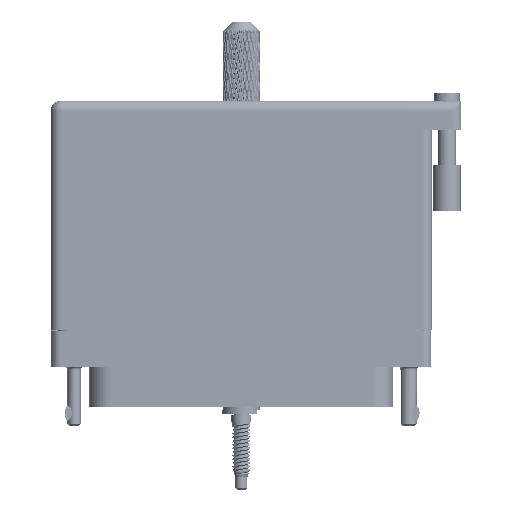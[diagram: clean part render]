
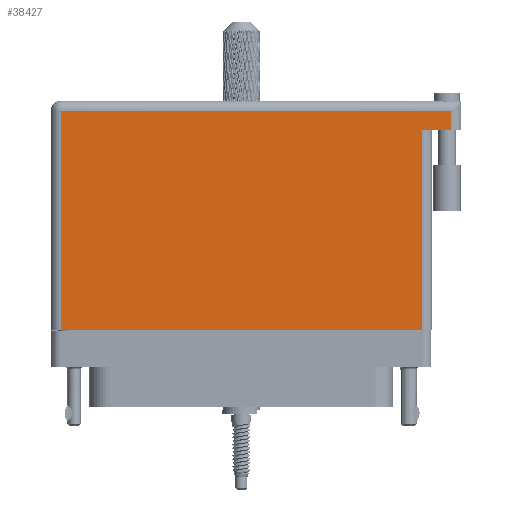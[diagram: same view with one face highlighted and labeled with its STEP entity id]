
A CAD part, front view. The second image highlights one B-rep face of the part: STEP entity #38427.
In plain terms, the highlighted face is planar.
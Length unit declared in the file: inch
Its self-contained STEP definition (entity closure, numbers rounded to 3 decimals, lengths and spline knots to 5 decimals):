
#741 = DIRECTION ( 'NONE',  ( -1., 0., 0. ) ) ;
#2738 = CARTESIAN_POINT ( 'NONE',  ( 1.43, 1.396, 0.4495 ) ) ;
#4744 = VECTOR ( 'NONE', #31527, 39.37008 ) ;
#10670 = EDGE_CURVE ( 'NONE', #47260, #81781, #23073, .T. ) ;
#10924 = VECTOR ( 'NONE', #36004, 39.37008 ) ;
#16540 = DIRECTION ( 'NONE',  ( -1., 0., 0. ) ) ;
#17275 = EDGE_LOOP ( 'NONE', ( #55286, #59925, #31762, #42835, #38974, #119706 ) ) ;
#17758 = CARTESIAN_POINT ( 'NONE',  ( 1.5, 1.269, 0.4495 ) ) ;
#18884 = CARTESIAN_POINT ( 'NONE',  ( -1.23, -0.1, 0.4495 ) ) ;
#19882 = PLANE ( 'NONE',  #89633 ) ;
#21301 = LINE ( 'NONE', #60070, #81248 ) ;
#23073 = LINE ( 'NONE', #105219, #72124 ) ;
#27916 = VERTEX_POINT ( 'NONE', #2738 ) ;
#29138 = VECTOR ( 'NONE', #16540, 39.37008 ) ;
#30657 = LINE ( 'NONE', #42257, #4744 ) ;
#31527 = DIRECTION ( 'NONE',  ( 0., 1., 0. ) ) ;
#31762 = ORIENTED_EDGE ( 'NONE', *, *, #45868, .F. ) ;
#34643 = EDGE_CURVE ( 'NONE', #109111, #27916, #30657, .T. ) ;
#36004 = DIRECTION ( 'NONE',  ( -1., 0., 0. ) ) ;
#38427 = ADVANCED_FACE ( 'NONE', ( #98975 ), #19882, .F. ) ;
#38974 = ORIENTED_EDGE ( 'NONE', *, *, #100724, .T. ) ;
#42257 = CARTESIAN_POINT ( 'NONE',  ( 1.43, 1.466, 0.4495 ) ) ;
#42835 = ORIENTED_EDGE ( 'NONE', *, *, #34643, .T. ) ;
#45493 = CARTESIAN_POINT ( 'NONE',  ( -1.23, -0.1, 0.4495 ) ) ;
#45868 = EDGE_CURVE ( 'NONE', #109111, #75058, #55257, .T. ) ;
#47260 = VERTEX_POINT ( 'NONE', #45493 ) ;
#48550 = CARTESIAN_POINT ( 'NONE',  ( 1.23, 1.269, 0.4495 ) ) ;
#49439 = DIRECTION ( 'NONE',  ( 0., 0., -1. ) ) ;
#53772 = LINE ( 'NONE', #113964, #10924 ) ;
#55257 = LINE ( 'NONE', #17758, #29138 ) ;
#55286 = ORIENTED_EDGE ( 'NONE', *, *, #10670, .T. ) ;
#59925 = ORIENTED_EDGE ( 'NONE', *, *, #96136, .T. ) ;
#60070 = CARTESIAN_POINT ( 'NONE',  ( 1.23, 1.269, 0.4495 ) ) ;
#60246 = VERTEX_POINT ( 'NONE', #123441 ) ;
#66611 = LINE ( 'NONE', #18884, #94226 ) ;
#72124 = VECTOR ( 'NONE', #86352, 39.37008 ) ;
#75058 = VERTEX_POINT ( 'NONE', #48550 ) ;
#81248 = VECTOR ( 'NONE', #88474, 39.37008 ) ;
#81548 = CARTESIAN_POINT ( 'NONE',  ( 1.43, 1.269, 0.4495 ) ) ;
#81781 = VERTEX_POINT ( 'NONE', #92077 ) ;
#86080 = EDGE_CURVE ( 'NONE', #60246, #47260, #66611, .T. ) ;
#86352 = DIRECTION ( 'NONE',  ( 1., 0., 0. ) ) ;
#88474 = DIRECTION ( 'NONE',  ( 0., 1., 0. ) ) ;
#88475 = CARTESIAN_POINT ( 'NONE',  ( -1.3, 1.466, 0.4495 ) ) ;
#89633 = AXIS2_PLACEMENT_3D ( 'NONE', #88475, #49439, #741 ) ;
#92077 = CARTESIAN_POINT ( 'NONE',  ( 1.23, -0.1, 0.4495 ) ) ;
#94226 = VECTOR ( 'NONE', #108778, 39.37008 ) ;
#96136 = EDGE_CURVE ( 'NONE', #81781, #75058, #21301, .T. ) ;
#98975 = FACE_OUTER_BOUND ( 'NONE', #17275, .T. ) ;
#100724 = EDGE_CURVE ( 'NONE', #27916, #60246, #53772, .T. ) ;
#105219 = CARTESIAN_POINT ( 'NONE',  ( -1.3, -0.1, 0.4495 ) ) ;
#108778 = DIRECTION ( 'NONE',  ( 0., -1., 0. ) ) ;
#109111 = VERTEX_POINT ( 'NONE', #81548 ) ;
#113964 = CARTESIAN_POINT ( 'NONE',  ( -1.3, 1.396, 0.4495 ) ) ;
#119706 = ORIENTED_EDGE ( 'NONE', *, *, #86080, .T. ) ;
#123441 = CARTESIAN_POINT ( 'NONE',  ( -1.23, 1.396, 0.4495 ) ) ;
